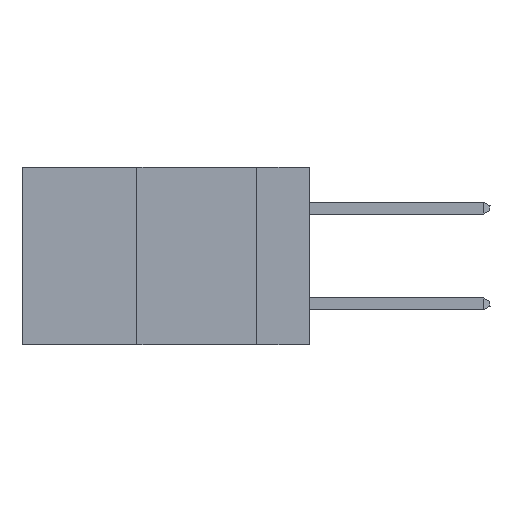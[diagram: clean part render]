
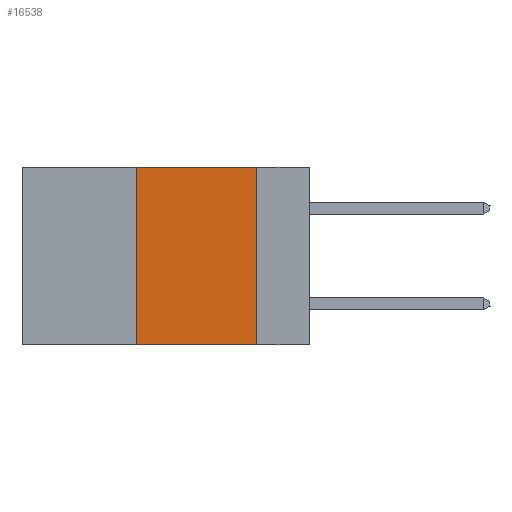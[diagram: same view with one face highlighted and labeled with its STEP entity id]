
A CAD part, left-side view. The second image highlights one B-rep face of the part: STEP entity #16538.
In plain terms, the highlighted planar face has unit normal (-1, 0, 0).
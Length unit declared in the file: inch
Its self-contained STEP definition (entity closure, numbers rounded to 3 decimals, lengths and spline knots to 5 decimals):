
#291 = ORIENTED_EDGE ( 'NONE', *, *, #31221, .F. ) ;
#1176 = CARTESIAN_POINT ( 'NONE',  ( 0., 0.36, 0. ) ) ;
#2430 = DIRECTION ( 'NONE',  ( 0., 0., -1. ) ) ;
#3208 = CARTESIAN_POINT ( 'NONE',  ( 0., 0.6, -0.37 ) ) ;
#3438 = CARTESIAN_POINT ( 'NONE',  ( 0., 0.6, 0. ) ) ;
#3772 = VERTEX_POINT ( 'NONE', #1176 ) ;
#4305 = CARTESIAN_POINT ( 'NONE',  ( 0., 0.6, 0. ) ) ;
#6895 = ORIENTED_EDGE ( 'NONE', *, *, #13487, .F. ) ;
#7143 = PLANE ( 'NONE',  #31538 ) ;
#9850 = LINE ( 'NONE', #3438, #23650 ) ;
#10431 = VECTOR ( 'NONE', #28044, 39.37008 ) ;
#13487 = EDGE_CURVE ( 'NONE', #3772, #34908, #9850, .T. ) ;
#13847 = LINE ( 'NONE', #29981, #20325 ) ;
#14588 = DIRECTION ( 'NONE',  ( 0., -1., 0. ) ) ;
#16538 = ADVANCED_FACE ( 'NONE', ( #34416 ), #7143, .F. ) ;
#16686 = CARTESIAN_POINT ( 'NONE',  ( 0., 0.36, 0. ) ) ;
#18238 = DIRECTION ( 'NONE',  ( 0., 0., -1. ) ) ;
#18453 = CARTESIAN_POINT ( 'NONE',  ( 0., 0.11, -0.37 ) ) ;
#19507 = DIRECTION ( 'NONE',  ( 0., 0., 1. ) ) ;
#20325 = VECTOR ( 'NONE', #2430, 39.37008 ) ;
#20667 = ORIENTED_EDGE ( 'NONE', *, *, #26462, .T. ) ;
#23043 = VECTOR ( 'NONE', #19507, 39.37008 ) ;
#23650 = VECTOR ( 'NONE', #14588, 39.37008 ) ;
#26462 = EDGE_CURVE ( 'NONE', #27913, #29184, #32266, .T. ) ;
#27185 = CARTESIAN_POINT ( 'NONE',  ( 0., 0.11, 0. ) ) ;
#27913 = VERTEX_POINT ( 'NONE', #31632 ) ;
#28044 = DIRECTION ( 'NONE',  ( 0., -1., 0. ) ) ;
#29184 = VERTEX_POINT ( 'NONE', #18453 ) ;
#29981 = CARTESIAN_POINT ( 'NONE',  ( 0., 0.11, 0. ) ) ;
#30258 = LINE ( 'NONE', #16686, #23043 ) ;
#31221 = EDGE_CURVE ( 'NONE', #34908, #29184, #13847, .T. ) ;
#31538 = AXIS2_PLACEMENT_3D ( 'NONE', #4305, #34547, #18238 ) ;
#31632 = CARTESIAN_POINT ( 'NONE',  ( 0., 0.36, -0.37 ) ) ;
#32176 = ORIENTED_EDGE ( 'NONE', *, *, #35542, .F. ) ;
#32266 = LINE ( 'NONE', #3208, #10431 ) ;
#33639 = EDGE_LOOP ( 'NONE', ( #291, #6895, #32176, #20667 ) ) ;
#34416 = FACE_OUTER_BOUND ( 'NONE', #33639, .T. ) ;
#34547 = DIRECTION ( 'NONE',  ( 1., 0., 0. ) ) ;
#34908 = VERTEX_POINT ( 'NONE', #27185 ) ;
#35542 = EDGE_CURVE ( 'NONE', #27913, #3772, #30258, .T. ) ;
